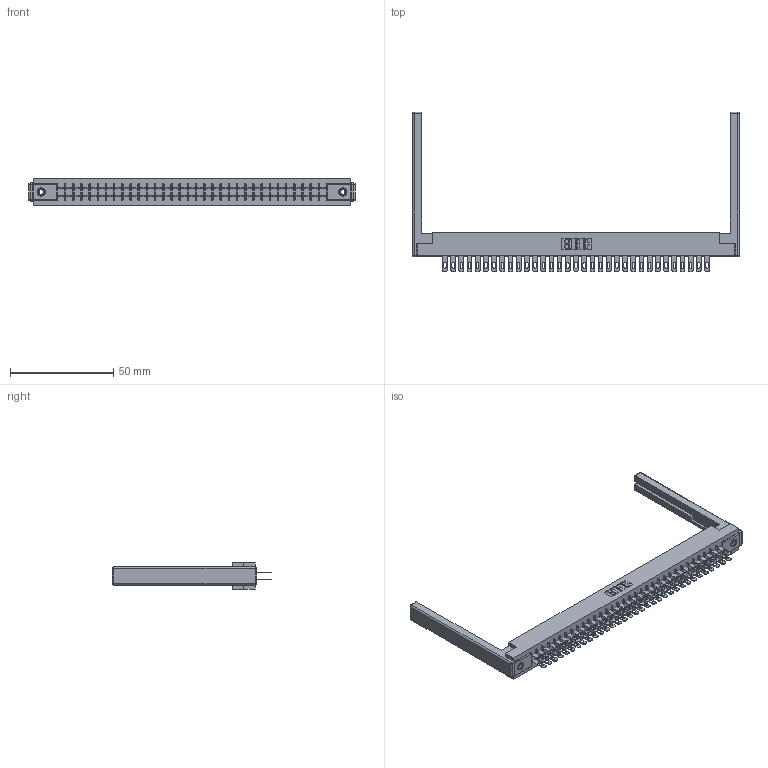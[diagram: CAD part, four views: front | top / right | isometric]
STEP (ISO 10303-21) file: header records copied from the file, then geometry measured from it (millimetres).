
FILE_DESCRIPTION (( 'STEP AP203' ), '1' );
FILE_NAME ('305-066-500-268.STEP', '2019-09-10T03:15:12', ( '' ), ( '' ), 'SwSTEP 2.0', 'SolidWorks 2016', '' );
FILE_SCHEMA (( 'CONFIG_CONTROL_DESIGN' ));
Length unit declared in the file: inch
Products named in the file (5): 305-290-001_500; 345-250-001_345-250-001-102; 305-066-500-268; 307-220-068; 305 Part_.156 Dia
Assembly tree (71 placements, depth 2):
  305-066-500-268
    305 Part_.156 Dia
    305-290-001_500  x66
    345-250-001_345-250-001-102  x2
    307-220-068  x2
Bounding box: 158.19 x 77.14 x 12.7 mm (x, y, z)
Volume: 21037.5 mm3; surface area: 26246.2 mm2
Topology: 71 solids, 71 shells, 3570 faces, 10177 edges, 6586 vertices
Faces by surface type: plane 2004, cylinder 1410, sphere 140, cone 12, torus 4
Entity records: 39607 total; most frequent: CARTESIAN_POINT 6526, ORIENTED_EDGE 6468, DIRECTION 6342, EDGE_CURVE 3234, VECTOR 2594, LINE 2594, VERTEX_POINT 2058, AXIS2_PLACEMENT_3D 1874
